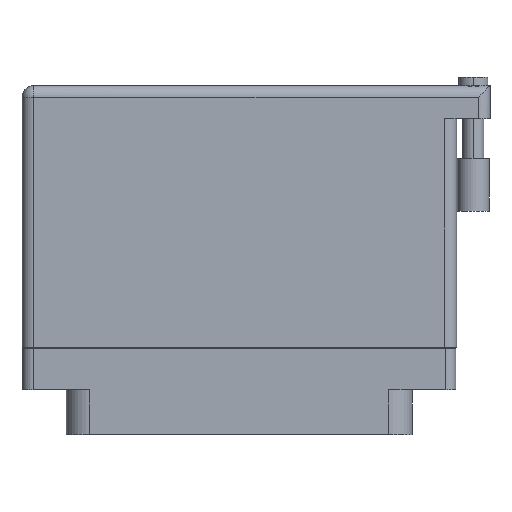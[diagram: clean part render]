
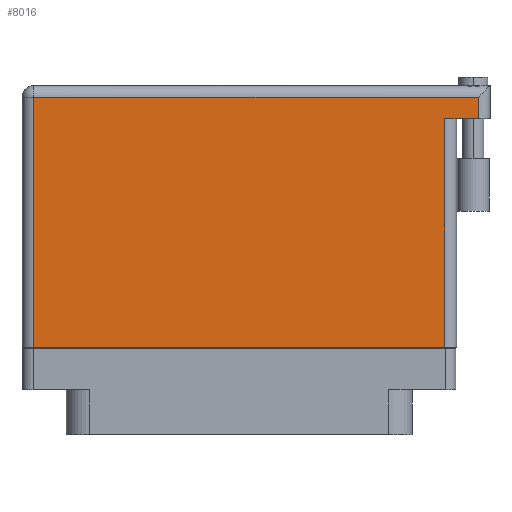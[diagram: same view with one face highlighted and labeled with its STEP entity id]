
A CAD part, front view. The second image highlights one B-rep face of the part: STEP entity #8016.
In plain terms, the highlighted face is planar.
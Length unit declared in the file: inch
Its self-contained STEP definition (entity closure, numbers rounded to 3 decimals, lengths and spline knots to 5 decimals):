
#160 = LINE ( 'NONE', #14853, #11076 ) ;
#240 = VECTOR ( 'NONE', #35898, 39.37008 ) ;
#975 = LINE ( 'NONE', #23607, #16360 ) ;
#1318 = LINE ( 'NONE', #12874, #7963 ) ;
#2383 = EDGE_LOOP ( 'NONE', ( #9905, #9617, #45220, #25971, #44105, #33255 ) ) ;
#2552 = CARTESIAN_POINT ( 'NONE',  ( 1.43, 1.396, 0.4495 ) ) ;
#4604 = VERTEX_POINT ( 'NONE', #2552 ) ;
#5231 = VERTEX_POINT ( 'NONE', #19956 ) ;
#6870 = CARTESIAN_POINT ( 'NONE',  ( 1.23, 1.269, 0.4495 ) ) ;
#7015 = CARTESIAN_POINT ( 'NONE',  ( -1.3, 1.396, 0.4495 ) ) ;
#7343 = DIRECTION ( 'NONE',  ( 0., 1., 0. ) ) ;
#7963 = VECTOR ( 'NONE', #8784, 39.37008 ) ;
#8016 = ADVANCED_FACE ( 'NONE', ( #46728 ), #28690, .F. ) ;
#8271 = AXIS2_PLACEMENT_3D ( 'NONE', #43133, #43358, #10401 ) ;
#8413 = VECTOR ( 'NONE', #7343, 39.37008 ) ;
#8784 = DIRECTION ( 'NONE',  ( 0., -1., 0. ) ) ;
#9617 = ORIENTED_EDGE ( 'NONE', *, *, #37279, .T. ) ;
#9905 = ORIENTED_EDGE ( 'NONE', *, *, #15514, .T. ) ;
#10392 = LINE ( 'NONE', #7015, #240 ) ;
#10401 = DIRECTION ( 'NONE',  ( -1., 0., 0. ) ) ;
#11076 = VECTOR ( 'NONE', #29520, 39.37008 ) ;
#12002 = DIRECTION ( 'NONE',  ( -1., 0., 0. ) ) ;
#12874 = CARTESIAN_POINT ( 'NONE',  ( -1.23, -0.1, 0.4495 ) ) ;
#13559 = EDGE_CURVE ( 'NONE', #21472, #4604, #975, .T. ) ;
#14853 = CARTESIAN_POINT ( 'NONE',  ( -1.3, -0.1, 0.4495 ) ) ;
#14863 = CARTESIAN_POINT ( 'NONE',  ( -1.23, 1.396, 0.4495 ) ) ;
#15514 = EDGE_CURVE ( 'NONE', #5231, #28518, #160, .T. ) ;
#16360 = VECTOR ( 'NONE', #19050, 39.37008 ) ;
#19050 = DIRECTION ( 'NONE',  ( 0., 1., 0. ) ) ;
#19956 = CARTESIAN_POINT ( 'NONE',  ( -1.23, -0.1, 0.4495 ) ) ;
#20667 = VECTOR ( 'NONE', #12002, 39.37008 ) ;
#21472 = VERTEX_POINT ( 'NONE', #42845 ) ;
#23607 = CARTESIAN_POINT ( 'NONE',  ( 1.43, 1.466, 0.4495 ) ) ;
#25840 = EDGE_CURVE ( 'NONE', #46485, #5231, #1318, .T. ) ;
#25971 = ORIENTED_EDGE ( 'NONE', *, *, #13559, .T. ) ;
#28518 = VERTEX_POINT ( 'NONE', #42048 ) ;
#28690 = PLANE ( 'NONE',  #8271 ) ;
#29520 = DIRECTION ( 'NONE',  ( 1., 0., 0. ) ) ;
#32391 = LINE ( 'NONE', #6870, #8413 ) ;
#32533 = EDGE_CURVE ( 'NONE', #21472, #43473, #44963, .T. ) ;
#33255 = ORIENTED_EDGE ( 'NONE', *, *, #25840, .T. ) ;
#35898 = DIRECTION ( 'NONE',  ( -1., 0., 0. ) ) ;
#37279 = EDGE_CURVE ( 'NONE', #28518, #43473, #32391, .T. ) ;
#38222 = CARTESIAN_POINT ( 'NONE',  ( 1.5, 1.269, 0.4495 ) ) ;
#38228 = CARTESIAN_POINT ( 'NONE',  ( 1.23, 1.269, 0.4495 ) ) ;
#40702 = EDGE_CURVE ( 'NONE', #4604, #46485, #10392, .T. ) ;
#42048 = CARTESIAN_POINT ( 'NONE',  ( 1.23, -0.1, 0.4495 ) ) ;
#42845 = CARTESIAN_POINT ( 'NONE',  ( 1.43, 1.269, 0.4495 ) ) ;
#43133 = CARTESIAN_POINT ( 'NONE',  ( -1.3, 1.466, 0.4495 ) ) ;
#43358 = DIRECTION ( 'NONE',  ( 0., 0., -1. ) ) ;
#43473 = VERTEX_POINT ( 'NONE', #38228 ) ;
#44105 = ORIENTED_EDGE ( 'NONE', *, *, #40702, .T. ) ;
#44963 = LINE ( 'NONE', #38222, #20667 ) ;
#45220 = ORIENTED_EDGE ( 'NONE', *, *, #32533, .F. ) ;
#46485 = VERTEX_POINT ( 'NONE', #14863 ) ;
#46728 = FACE_OUTER_BOUND ( 'NONE', #2383, .T. ) ;
